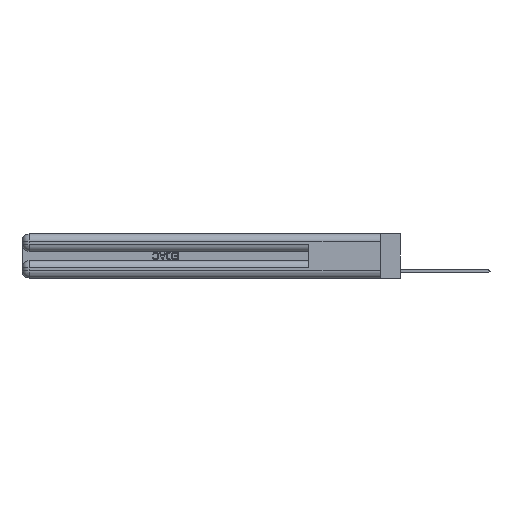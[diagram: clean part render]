
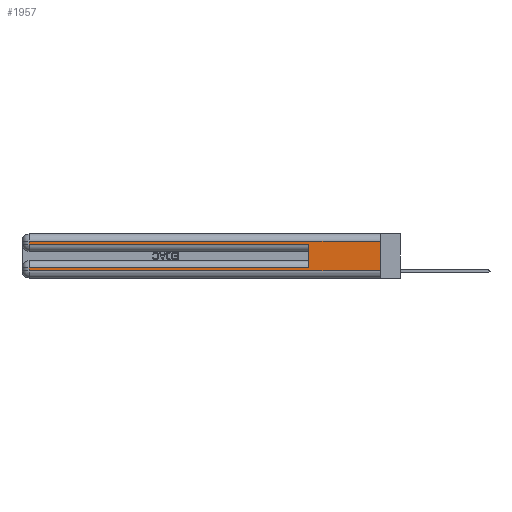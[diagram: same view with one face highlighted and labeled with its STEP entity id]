
A CAD part, left-side view. The second image highlights one B-rep face of the part: STEP entity #1957.
In plain terms, the highlighted planar face has unit normal (-1, 0, 0).
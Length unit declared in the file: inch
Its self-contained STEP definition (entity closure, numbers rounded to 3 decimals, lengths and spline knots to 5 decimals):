
#4 = VECTOR ( 'NONE', #19331, 39.37008 ) ;
#295 = CARTESIAN_POINT ( 'NONE',  ( 0., 0., 0.31 ) ) ;
#659 = ORIENTED_EDGE ( 'NONE', *, *, #3553, .T. ) ;
#973 = CARTESIAN_POINT ( 'NONE',  ( 0., 0.6, 0.085 ) ) ;
#1598 = DIRECTION ( 'NONE',  ( 0., 0., -1. ) ) ;
#1727 = VECTOR ( 'NONE', #15828, 39.37008 ) ;
#1824 = CARTESIAN_POINT ( 'NONE',  ( 0., 0., 0.06 ) ) ;
#1957 = ADVANCED_FACE ( 'NONE', ( #19697 ), #28570, .F. ) ;
#2244 = ORIENTED_EDGE ( 'NONE', *, *, #23049, .T. ) ;
#3553 = EDGE_CURVE ( 'NONE', #18395, #13212, #19618, .T. ) ;
#3883 = CARTESIAN_POINT ( 'NONE',  ( 0., 2.94, 0.37 ) ) ;
#4331 = EDGE_LOOP ( 'NONE', ( #23468, #10408, #27786, #24633, #24996, #2244, #659, #24971 ) ) ;
#4338 = EDGE_CURVE ( 'NONE', #28493, #11535, #10781, .T. ) ;
#4848 = VECTOR ( 'NONE', #17344, 39.37008 ) ;
#5200 = VECTOR ( 'NONE', #19442, 39.37008 ) ;
#5388 = CARTESIAN_POINT ( 'NONE',  ( 0., 0.6, 0.285 ) ) ;
#5479 = VECTOR ( 'NONE', #22026, 39.37008 ) ;
#5611 = CARTESIAN_POINT ( 'NONE',  ( 0., 2.94, 0.31 ) ) ;
#5858 = LINE ( 'NONE', #28599, #4 ) ;
#5980 = CARTESIAN_POINT ( 'NONE',  ( 0., 0., 0.37 ) ) ;
#6287 = VERTEX_POINT ( 'NONE', #5611 ) ;
#7292 = CARTESIAN_POINT ( 'NONE',  ( 0., 0., 0.37 ) ) ;
#8694 = LINE ( 'NONE', #14970, #5200 ) ;
#9393 = VECTOR ( 'NONE', #20575, 39.37008 ) ;
#10408 = ORIENTED_EDGE ( 'NONE', *, *, #13611, .T. ) ;
#10781 = LINE ( 'NONE', #17522, #5479 ) ;
#11535 = VERTEX_POINT ( 'NONE', #5388 ) ;
#11988 = VERTEX_POINT ( 'NONE', #24704 ) ;
#12893 = LINE ( 'NONE', #7292, #9393 ) ;
#12898 = EDGE_CURVE ( 'NONE', #15861, #11535, #5858, .T. ) ;
#13212 = VERTEX_POINT ( 'NONE', #19758 ) ;
#13433 = EDGE_CURVE ( 'NONE', #13212, #11988, #24809, .T. ) ;
#13611 = EDGE_CURVE ( 'NONE', #24676, #6287, #16399, .T. ) ;
#13944 = CARTESIAN_POINT ( 'NONE',  ( 0., 0., 0.31 ) ) ;
#14666 = LINE ( 'NONE', #3883, #4848 ) ;
#14928 = CARTESIAN_POINT ( 'NONE',  ( 0., 2.94, 0.37 ) ) ;
#14970 = CARTESIAN_POINT ( 'NONE',  ( 0., 0., 0.085 ) ) ;
#15522 = CARTESIAN_POINT ( 'NONE',  ( 0., 2.94, 0.285 ) ) ;
#15740 = AXIS2_PLACEMENT_3D ( 'NONE', #5980, #26197, #24245 ) ;
#15828 = DIRECTION ( 'NONE',  ( 0., 1., 0. ) ) ;
#15861 = VERTEX_POINT ( 'NONE', #15522 ) ;
#16399 = LINE ( 'NONE', #13944, #1727 ) ;
#17344 = DIRECTION ( 'NONE',  ( 0., 0., -1. ) ) ;
#17522 = CARTESIAN_POINT ( 'NONE',  ( 0., 0.6, 0.145 ) ) ;
#18395 = VERTEX_POINT ( 'NONE', #28323 ) ;
#18880 = EDGE_CURVE ( 'NONE', #6287, #15861, #14666, .T. ) ;
#19331 = DIRECTION ( 'NONE',  ( 0., -1., 0. ) ) ;
#19442 = DIRECTION ( 'NONE',  ( 0., 1., 0. ) ) ;
#19618 = LINE ( 'NONE', #14928, #20327 ) ;
#19697 = FACE_OUTER_BOUND ( 'NONE', #4331, .T. ) ;
#19758 = CARTESIAN_POINT ( 'NONE',  ( 0., 2.94, 0.06 ) ) ;
#20327 = VECTOR ( 'NONE', #1598, 39.37008 ) ;
#20575 = DIRECTION ( 'NONE',  ( 0., 0., -1. ) ) ;
#22026 = DIRECTION ( 'NONE',  ( 0., 0., 1. ) ) ;
#23049 = EDGE_CURVE ( 'NONE', #28493, #18395, #8694, .T. ) ;
#23468 = ORIENTED_EDGE ( 'NONE', *, *, #27527, .F. ) ;
#24043 = DIRECTION ( 'NONE',  ( 0., -1., 0. ) ) ;
#24112 = VECTOR ( 'NONE', #24043, 39.37008 ) ;
#24245 = DIRECTION ( 'NONE',  ( 0., 0., -1. ) ) ;
#24633 = ORIENTED_EDGE ( 'NONE', *, *, #12898, .T. ) ;
#24676 = VERTEX_POINT ( 'NONE', #295 ) ;
#24704 = CARTESIAN_POINT ( 'NONE',  ( 0., 0., 0.06 ) ) ;
#24809 = LINE ( 'NONE', #1824, #24112 ) ;
#24971 = ORIENTED_EDGE ( 'NONE', *, *, #13433, .T. ) ;
#24996 = ORIENTED_EDGE ( 'NONE', *, *, #4338, .F. ) ;
#26197 = DIRECTION ( 'NONE',  ( 1., 0., 0. ) ) ;
#27527 = EDGE_CURVE ( 'NONE', #24676, #11988, #12893, .T. ) ;
#27786 = ORIENTED_EDGE ( 'NONE', *, *, #18880, .T. ) ;
#28323 = CARTESIAN_POINT ( 'NONE',  ( 0., 2.94, 0.085 ) ) ;
#28493 = VERTEX_POINT ( 'NONE', #973 ) ;
#28570 = PLANE ( 'NONE',  #15740 ) ;
#28599 = CARTESIAN_POINT ( 'NONE',  ( 0., 0., 0.285 ) ) ;
